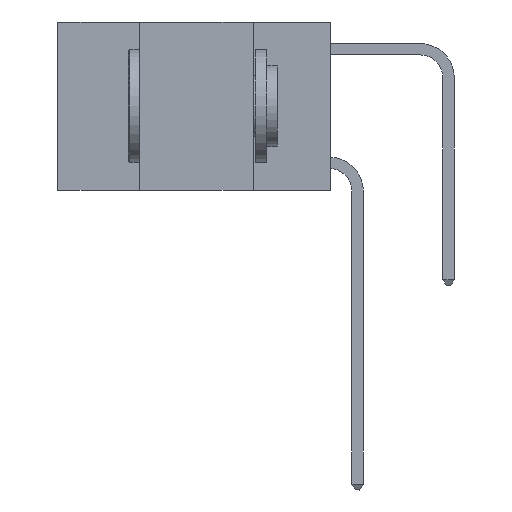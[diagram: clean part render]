
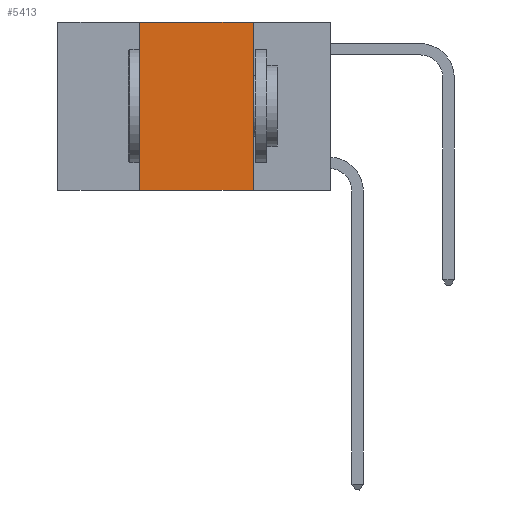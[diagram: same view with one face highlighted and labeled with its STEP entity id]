
A CAD part, left-side view. The second image highlights one B-rep face of the part: STEP entity #5413.
In plain terms, the highlighted planar face has unit normal (-1, 0, 0).
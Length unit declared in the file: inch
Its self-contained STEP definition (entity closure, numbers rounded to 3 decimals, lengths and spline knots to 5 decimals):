
#313 = LINE ( 'NONE', #6907, #9680 ) ;
#2300 = CARTESIAN_POINT ( 'NONE',  ( 0., 0.6, 0. ) ) ;
#2489 = ORIENTED_EDGE ( 'NONE', *, *, #27056, .F. ) ;
#2612 = VERTEX_POINT ( 'NONE', #6666 ) ;
#4127 = EDGE_CURVE ( 'NONE', #2612, #24020, #19611, .T. ) ;
#4660 = VERTEX_POINT ( 'NONE', #4782 ) ;
#4782 = CARTESIAN_POINT ( 'NONE',  ( 0., 0.42, 0. ) ) ;
#5413 = ADVANCED_FACE ( 'NONE', ( #6964 ), #6678, .F. ) ;
#6666 = CARTESIAN_POINT ( 'NONE',  ( 0., 0.42, -0.37 ) ) ;
#6678 = PLANE ( 'NONE',  #7593 ) ;
#6907 = CARTESIAN_POINT ( 'NONE',  ( 0., 0.42, 0. ) ) ;
#6964 = FACE_OUTER_BOUND ( 'NONE', #16975, .T. ) ;
#7226 = DIRECTION ( 'NONE',  ( 0., 0., -1. ) ) ;
#7593 = AXIS2_PLACEMENT_3D ( 'NONE', #24199, #15718, #24482 ) ;
#8923 = DIRECTION ( 'NONE',  ( 0., 0., 1. ) ) ;
#9680 = VECTOR ( 'NONE', #8923, 39.37008 ) ;
#9902 = EDGE_CURVE ( 'NONE', #2612, #4660, #313, .T. ) ;
#10040 = CARTESIAN_POINT ( 'NONE',  ( 0., 0.17, 0. ) ) ;
#10710 = VECTOR ( 'NONE', #26198, 39.37008 ) ;
#11043 = VECTOR ( 'NONE', #24273, 39.37008 ) ;
#15274 = CARTESIAN_POINT ( 'NONE',  ( 0., 0.6, -0.37 ) ) ;
#15360 = LINE ( 'NONE', #2300, #11043 ) ;
#15479 = EDGE_CURVE ( 'NONE', #4660, #19000, #15360, .T. ) ;
#15718 = DIRECTION ( 'NONE',  ( 1., 0., 0. ) ) ;
#16382 = ORIENTED_EDGE ( 'NONE', *, *, #15479, .F. ) ;
#16975 = EDGE_LOOP ( 'NONE', ( #2489, #16382, #24314, #25422 ) ) ;
#19000 = VERTEX_POINT ( 'NONE', #10040 ) ;
#19611 = LINE ( 'NONE', #15274, #10710 ) ;
#23746 = VECTOR ( 'NONE', #7226, 39.37008 ) ;
#24020 = VERTEX_POINT ( 'NONE', #27061 ) ;
#24199 = CARTESIAN_POINT ( 'NONE',  ( 0., 0.6, 0. ) ) ;
#24273 = DIRECTION ( 'NONE',  ( 0., -1., 0. ) ) ;
#24314 = ORIENTED_EDGE ( 'NONE', *, *, #9902, .F. ) ;
#24465 = LINE ( 'NONE', #26756, #23746 ) ;
#24482 = DIRECTION ( 'NONE',  ( 0., 0., -1. ) ) ;
#25422 = ORIENTED_EDGE ( 'NONE', *, *, #4127, .T. ) ;
#26198 = DIRECTION ( 'NONE',  ( 0., -1., 0. ) ) ;
#26756 = CARTESIAN_POINT ( 'NONE',  ( 0., 0.17, 0. ) ) ;
#27056 = EDGE_CURVE ( 'NONE', #19000, #24020, #24465, .T. ) ;
#27061 = CARTESIAN_POINT ( 'NONE',  ( 0., 0.17, -0.37 ) ) ;
